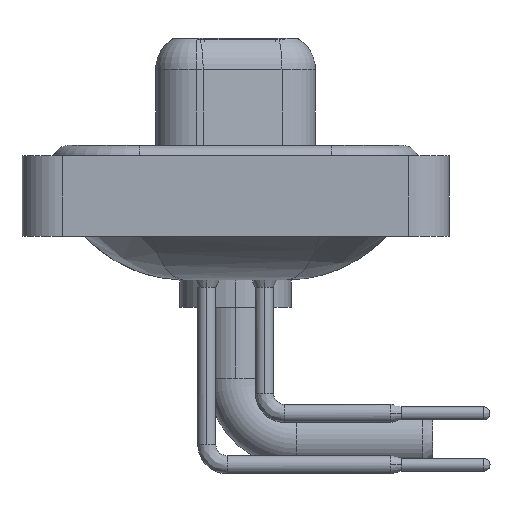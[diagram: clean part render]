
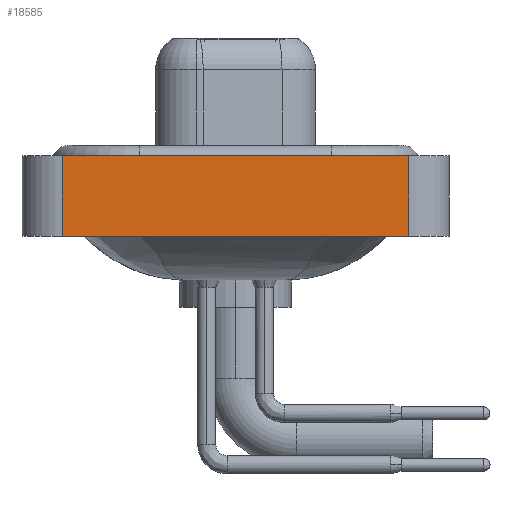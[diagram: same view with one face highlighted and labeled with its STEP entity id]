
A CAD part, left-side view. The second image highlights one B-rep face of the part: STEP entity #18585.
In plain terms, the highlighted planar face has unit normal (-1, 0, 0).
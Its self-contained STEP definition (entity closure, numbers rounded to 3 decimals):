
#300 = DIRECTION ( 'NONE',  ( 0., -1., 0. ) ) ;
#509 = CARTESIAN_POINT ( 'NONE',  ( -7.25, -8.55, -3.6 ) ) ;
#678 = LINE ( 'NONE', #2090, #16463 ) ;
#2090 = CARTESIAN_POINT ( 'NONE',  ( -7.25, 8.55, -3.6 ) ) ;
#2181 = VECTOR ( 'NONE', #15232, 1000. ) ;
#2182 = VECTOR ( 'NONE', #300, 1000. ) ;
#2692 = CARTESIAN_POINT ( 'NONE',  ( -7.25, -8.55, 0.4 ) ) ;
#2897 = ORIENTED_EDGE ( 'NONE', *, *, #6438, .T. ) ;
#3086 = DIRECTION ( 'NONE',  ( -1., 0., 0. ) ) ;
#3523 = CARTESIAN_POINT ( 'NONE',  ( -7.25, 8.55, -3.6 ) ) ;
#5918 = CARTESIAN_POINT ( 'NONE',  ( -7.25, -8.55, -3.6 ) ) ;
#6226 = DIRECTION ( 'NONE',  ( 0., 0., 1. ) ) ;
#6438 = EDGE_CURVE ( 'NONE', #10461, #15591, #18944, .T. ) ;
#6502 = CARTESIAN_POINT ( 'NONE',  ( -7.25, -8.55, -3.6 ) ) ;
#6620 = AXIS2_PLACEMENT_3D ( 'NONE', #5918, #3086, #6226 ) ;
#7398 = ORIENTED_EDGE ( 'NONE', *, *, #14645, .T. ) ;
#7590 = CARTESIAN_POINT ( 'NONE',  ( -7.25, -8.55, -3.6 ) ) ;
#7945 = VERTEX_POINT ( 'NONE', #3523 ) ;
#8055 = VERTEX_POINT ( 'NONE', #17715 ) ;
#8595 = EDGE_CURVE ( 'NONE', #7945, #8055, #678, .T. ) ;
#9142 = PLANE ( 'NONE',  #6620 ) ;
#10461 = VERTEX_POINT ( 'NONE', #6502 ) ;
#11069 = LINE ( 'NONE', #15673, #2182 ) ;
#12226 = ORIENTED_EDGE ( 'NONE', *, *, #8595, .F. ) ;
#12270 = FACE_OUTER_BOUND ( 'NONE', #16660, .T. ) ;
#12421 = DIRECTION ( 'NONE',  ( 0., 0., 1. ) ) ;
#14645 = EDGE_CURVE ( 'NONE', #7945, #10461, #19656, .T. ) ;
#15232 = DIRECTION ( 'NONE',  ( 0., -1., 0. ) ) ;
#15462 = ORIENTED_EDGE ( 'NONE', *, *, #17178, .F. ) ;
#15591 = VERTEX_POINT ( 'NONE', #2692 ) ;
#15673 = CARTESIAN_POINT ( 'NONE',  ( -7.25, -8.55, 0.4 ) ) ;
#16079 = DIRECTION ( 'NONE',  ( 0., 0., 1. ) ) ;
#16463 = VECTOR ( 'NONE', #16079, 1000. ) ;
#16660 = EDGE_LOOP ( 'NONE', ( #2897, #15462, #12226, #7398 ) ) ;
#17178 = EDGE_CURVE ( 'NONE', #8055, #15591, #11069, .T. ) ;
#17715 = CARTESIAN_POINT ( 'NONE',  ( -7.25, 8.55, 0.4 ) ) ;
#18585 = ADVANCED_FACE ( 'NONE', ( #12270 ), #9142, .T. ) ;
#18944 = LINE ( 'NONE', #509, #19365 ) ;
#19365 = VECTOR ( 'NONE', #12421, 1000. ) ;
#19656 = LINE ( 'NONE', #7590, #2181 ) ;
